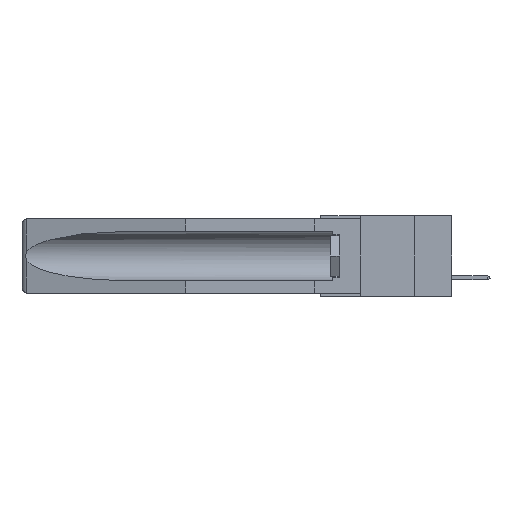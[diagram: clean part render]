
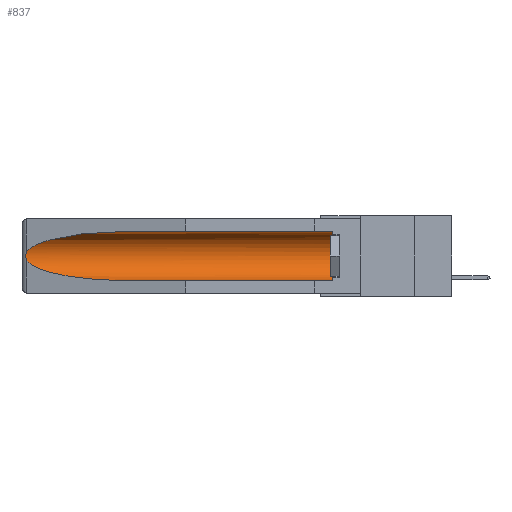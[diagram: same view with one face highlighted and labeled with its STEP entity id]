
A CAD part, left-side view. The second image highlights one B-rep face of the part: STEP entity #837.
In plain terms, the highlighted cylindrical face has radius 2.857 mm (diameter 5.715 mm), a partial arc.
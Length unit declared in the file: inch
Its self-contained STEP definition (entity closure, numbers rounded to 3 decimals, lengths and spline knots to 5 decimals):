
#104 = DIRECTION ( 'NONE',  ( 0., -1., 0. ) ) ;
#409 = FACE_OUTER_BOUND ( 'NONE', #9087, .T. ) ;
#837 = ADVANCED_FACE ( 'NONE', ( #409 ), #6902, .F. ) ;
#1086 = VERTEX_POINT ( 'NONE', #9066 ) ;
#1192 = DIRECTION ( 'NONE',  ( 0., 1., 0. ) ) ;
#1206 = CARTESIAN_POINT ( 'NONE',  ( 0.155, 1.07973, -0.284 ) ) ;
#1352 = CARTESIAN_POINT ( 'NONE',  ( 0.155, 0.126, -0.284 ) ) ;
#2058 = CARTESIAN_POINT ( 'NONE',  ( 0.2675, 1.53308, -0.17534 ) ) ;
#2152 = VERTEX_POINT ( 'NONE', #3518 ) ;
#2595 = LINE ( 'NONE', #7092, #18095 ) ;
#2695 = CARTESIAN_POINT ( 'NONE',  ( 0.25451, 1.48313, -0.24835 ) ) ;
#2733 = VERTEX_POINT ( 'NONE', #9989 ) ;
#3518 = CARTESIAN_POINT ( 'NONE',  ( 0.26537, 1.52718, -0.19328 ) ) ;
#4218 = CARTESIAN_POINT ( 'NONE',  ( 0.26537, 1.52718, -0.19328 ) ) ;
#4535 = EDGE_CURVE ( 'NONE', #2152, #19119, #11121, .T. ) ;
#5005 = CARTESIAN_POINT ( 'NONE',  ( 0.26537, 1.52718, -0.14972 ) ) ;
#5011 = CARTESIAN_POINT ( 'NONE',  ( 0.2673, 1.53269, -0.17917 ) ) ;
#5185 = ORIENTED_EDGE ( 'NONE', *, *, #6771, .T. ) ;
#5899 = AXIS2_PLACEMENT_3D ( 'NONE', #17836, #104, #13426 ) ;
#6455 = CARTESIAN_POINT ( 'NONE',  ( 0.21114, 1.30732, -0.059 ) ) ;
#6460 = CARTESIAN_POINT ( 'NONE',  ( 0.2673, 1.5327, -0.16383 ) ) ;
#6771 = EDGE_CURVE ( 'NONE', #14957, #1086, #8529, .T. ) ;
#6902 = CYLINDRICAL_SURFACE ( 'NONE', #19013, 0.1125 ) ;
#7092 = CARTESIAN_POINT ( 'NONE',  ( 0.155, -0.30754, -0.059 ) ) ;
#7821 = EDGE_CURVE ( 'NONE', #1086, #2152, #15028, .T. ) ;
#8013 = CARTESIAN_POINT ( 'NONE',  ( 0.2675, 1.53308, -0.16763 ) ) ;
#8428 = ORIENTED_EDGE ( 'NONE', *, *, #7821, .T. ) ;
#8529 =( BOUNDED_CURVE ( )  B_SPLINE_CURVE ( 3, ( #18468, #6455, #15489, #5005 ),
 .UNSPECIFIED., .F., .F. ) 
 B_SPLINE_CURVE_WITH_KNOTS ( ( 4, 4 ),
 ( 4.71239, 6.08839 ),
 .UNSPECIFIED. ) 
 CURVE ( )  GEOMETRIC_REPRESENTATION_ITEM ( )  RATIONAL_B_SPLINE_CURVE ( ( 1., 0.848, 0.848, 1. ) ) 
 REPRESENTATION_ITEM ( '' )  );
#9066 = CARTESIAN_POINT ( 'NONE',  ( 0.26537, 1.52718, -0.14972 ) ) ;
#9087 = EDGE_LOOP ( 'NONE', ( #5185, #8428, #17017, #14294, #19145, #11712 ) ) ;
#9433 = CARTESIAN_POINT ( 'NONE',  ( 0.26537, 1.52718, -0.19328 ) ) ;
#9603 = DIRECTION ( 'NONE',  ( 0., 1., 0. ) ) ;
#9989 = CARTESIAN_POINT ( 'NONE',  ( 0.155, 0.126, -0.059 ) ) ;
#10740 = CIRCLE ( 'NONE', #5899, 0.1125 ) ;
#10795 = CARTESIAN_POINT ( 'NONE',  ( 0.26597, 1.52961, -0.15275 ) ) ;
#10859 = CARTESIAN_POINT ( 'NONE',  ( 0.155, -0.30754, -0.1715 ) ) ;
#10915 = DIRECTION ( 'NONE',  ( 0., 0., 1. ) ) ;
#11121 =( BOUNDED_CURVE ( )  B_SPLINE_CURVE ( 3, ( #4218, #2695, #14516, #16254 ),
 .UNSPECIFIED., .F., .F. ) 
 B_SPLINE_CURVE_WITH_KNOTS ( ( 4, 4 ),
 ( 0.1948, 1.5708 ),
 .UNSPECIFIED. ) 
 CURVE ( )  GEOMETRIC_REPRESENTATION_ITEM ( )  RATIONAL_B_SPLINE_CURVE ( ( 1., 0.848, 0.848, 1. ) ) 
 REPRESENTATION_ITEM ( '' )  );
#11712 = ORIENTED_EDGE ( 'NONE', *, *, #15935, .T. ) ;
#12126 = VECTOR ( 'NONE', #12771, 39.37008 ) ;
#12521 = CARTESIAN_POINT ( 'NONE',  ( 0.26597, 1.5296, -0.19026 ) ) ;
#12771 = DIRECTION ( 'NONE',  ( 0., 1., 0. ) ) ;
#13426 = DIRECTION ( 'NONE',  ( 0., 0., 1. ) ) ;
#14013 = CARTESIAN_POINT ( 'NONE',  ( 0.26655, 1.53094, -0.18657 ) ) ;
#14254 = VERTEX_POINT ( 'NONE', #1352 ) ;
#14294 = ORIENTED_EDGE ( 'NONE', *, *, #17978, .F. ) ;
#14489 = EDGE_CURVE ( 'NONE', #14254, #2733, #10740, .T. ) ;
#14516 = CARTESIAN_POINT ( 'NONE',  ( 0.21114, 1.30732, -0.284 ) ) ;
#14957 = VERTEX_POINT ( 'NONE', #16322 ) ;
#15028 = B_SPLINE_CURVE_WITH_KNOTS ( 'NONE', 3,
 ( #18159, #10795, #18536, #6460, #8013, #2058, #5011, #14013, #12521, #9433 ),
 .UNSPECIFIED., .F., .F.,
 ( 4, 2, 2, 2, 4 ),
 ( 0., 0.00029, 0.00058, 0.00087, 0.00117 ),
 .UNSPECIFIED. ) ;
#15489 = CARTESIAN_POINT ( 'NONE',  ( 0.25451, 1.48313, -0.09465 ) ) ;
#15935 = EDGE_CURVE ( 'NONE', #2733, #14957, #2595, .T. ) ;
#16254 = CARTESIAN_POINT ( 'NONE',  ( 0.155, 1.07973, -0.284 ) ) ;
#16322 = CARTESIAN_POINT ( 'NONE',  ( 0.155, 1.07973, -0.059 ) ) ;
#16959 = CARTESIAN_POINT ( 'NONE',  ( 0.155, -0.30754, -0.284 ) ) ;
#17017 = ORIENTED_EDGE ( 'NONE', *, *, #4535, .T. ) ;
#17183 = LINE ( 'NONE', #16959, #12126 ) ;
#17836 = CARTESIAN_POINT ( 'NONE',  ( 0.155, 0.126, -0.1715 ) ) ;
#17978 = EDGE_CURVE ( 'NONE', #14254, #19119, #17183, .T. ) ;
#18095 = VECTOR ( 'NONE', #1192, 39.37008 ) ;
#18159 = CARTESIAN_POINT ( 'NONE',  ( 0.26537, 1.52718, -0.14972 ) ) ;
#18468 = CARTESIAN_POINT ( 'NONE',  ( 0.155, 1.07973, -0.059 ) ) ;
#18536 = CARTESIAN_POINT ( 'NONE',  ( 0.26654, 1.53092, -0.15636 ) ) ;
#19013 = AXIS2_PLACEMENT_3D ( 'NONE', #10859, #9603, #10915 ) ;
#19119 = VERTEX_POINT ( 'NONE', #1206 ) ;
#19145 = ORIENTED_EDGE ( 'NONE', *, *, #14489, .T. ) ;
